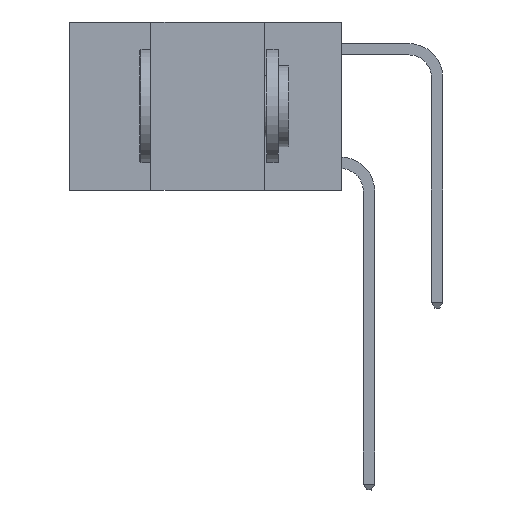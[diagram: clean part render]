
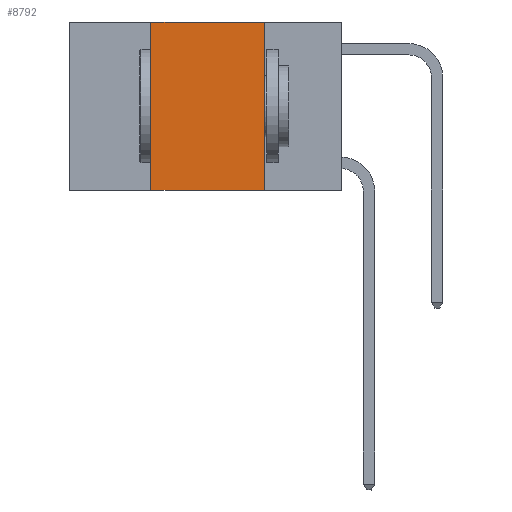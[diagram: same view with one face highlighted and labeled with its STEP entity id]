
A CAD part, left-side view. The second image highlights one B-rep face of the part: STEP entity #8792.
In plain terms, the highlighted planar face has unit normal (-1, 0, 0).
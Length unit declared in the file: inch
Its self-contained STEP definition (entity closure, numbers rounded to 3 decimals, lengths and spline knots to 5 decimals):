
#12 = CARTESIAN_POINT ( 'NONE',  ( 0., 0.42, 0. ) ) ;
#25 = VECTOR ( 'NONE', #6324, 39.37008 ) ;
#858 = EDGE_LOOP ( 'NONE', ( #9976, #6678, #4768, #7072 ) ) ;
#879 = VERTEX_POINT ( 'NONE', #12734 ) ;
#1125 = EDGE_CURVE ( 'NONE', #879, #7089, #12682, .T. ) ;
#2008 = VECTOR ( 'NONE', #6408, 39.37008 ) ;
#2716 = LINE ( 'NONE', #12723, #25 ) ;
#3776 = VERTEX_POINT ( 'NONE', #12 ) ;
#4447 = CARTESIAN_POINT ( 'NONE',  ( 0., 0.17, 0. ) ) ;
#4590 = VECTOR ( 'NONE', #7820, 39.37008 ) ;
#4768 = ORIENTED_EDGE ( 'NONE', *, *, #9614, .F. ) ;
#4903 = AXIS2_PLACEMENT_3D ( 'NONE', #9279, #11438, #4952 ) ;
#4952 = DIRECTION ( 'NONE',  ( 0., 0., -1. ) ) ;
#5817 = CARTESIAN_POINT ( 'NONE',  ( 0., 0.17, -0.37 ) ) ;
#6030 = PLANE ( 'NONE',  #4903 ) ;
#6324 = DIRECTION ( 'NONE',  ( 0., -1., 0. ) ) ;
#6408 = DIRECTION ( 'NONE',  ( 0., -1., 0. ) ) ;
#6657 = VECTOR ( 'NONE', #12202, 39.37008 ) ;
#6678 = ORIENTED_EDGE ( 'NONE', *, *, #7499, .F. ) ;
#7072 = ORIENTED_EDGE ( 'NONE', *, *, #12747, .T. ) ;
#7089 = VERTEX_POINT ( 'NONE', #5817 ) ;
#7219 = LINE ( 'NONE', #14166, #4590 ) ;
#7499 = EDGE_CURVE ( 'NONE', #3776, #879, #13607, .T. ) ;
#7820 = DIRECTION ( 'NONE',  ( 0., 0., 1. ) ) ;
#8792 = ADVANCED_FACE ( 'NONE', ( #11592 ), #6030, .F. ) ;
#9279 = CARTESIAN_POINT ( 'NONE',  ( 0., 0.6, 0. ) ) ;
#9614 = EDGE_CURVE ( 'NONE', #13693, #3776, #7219, .T. ) ;
#9976 = ORIENTED_EDGE ( 'NONE', *, *, #1125, .F. ) ;
#11438 = DIRECTION ( 'NONE',  ( 1., 0., 0. ) ) ;
#11592 = FACE_OUTER_BOUND ( 'NONE', #858, .T. ) ;
#11745 = CARTESIAN_POINT ( 'NONE',  ( 0., 0.6, 0. ) ) ;
#12202 = DIRECTION ( 'NONE',  ( 0., 0., -1. ) ) ;
#12682 = LINE ( 'NONE', #4447, #6657 ) ;
#12723 = CARTESIAN_POINT ( 'NONE',  ( 0., 0.6, -0.37 ) ) ;
#12734 = CARTESIAN_POINT ( 'NONE',  ( 0., 0.17, 0. ) ) ;
#12747 = EDGE_CURVE ( 'NONE', #13693, #7089, #2716, .T. ) ;
#13607 = LINE ( 'NONE', #11745, #2008 ) ;
#13693 = VERTEX_POINT ( 'NONE', #14058 ) ;
#14058 = CARTESIAN_POINT ( 'NONE',  ( 0., 0.42, -0.37 ) ) ;
#14166 = CARTESIAN_POINT ( 'NONE',  ( 0., 0.42, 0. ) ) ;
